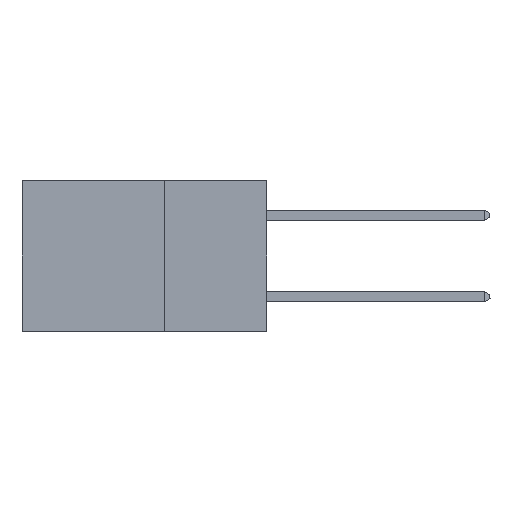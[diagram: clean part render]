
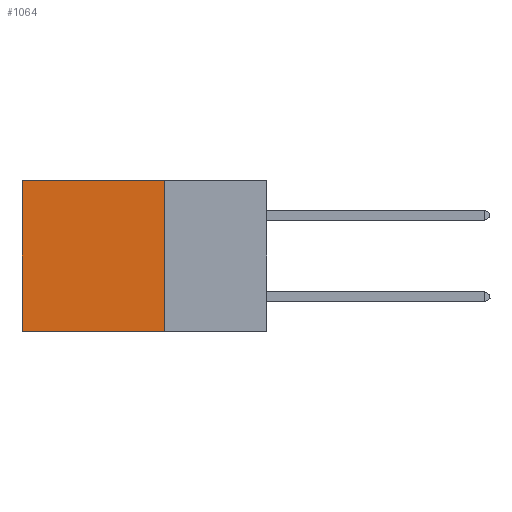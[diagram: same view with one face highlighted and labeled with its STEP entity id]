
A CAD part, left-side view. The second image highlights one B-rep face of the part: STEP entity #1064.
In plain terms, the highlighted planar face has unit normal (-1, 0, 0).
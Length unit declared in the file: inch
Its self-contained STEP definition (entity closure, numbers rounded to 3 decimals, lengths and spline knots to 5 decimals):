
#1064 = ADVANCED_FACE ( 'NONE', ( #12632 ), #14501, .F. ) ;
#1377 = ORIENTED_EDGE ( 'NONE', *, *, #7492, .T. ) ;
#2308 = DIRECTION ( 'NONE',  ( 0., 0., -1. ) ) ;
#2912 = CARTESIAN_POINT ( 'NONE',  ( 0.2875, 0.6, 0. ) ) ;
#4294 = DIRECTION ( 'NONE',  ( 0., 1., 0. ) ) ;
#4719 = VECTOR ( 'NONE', #12268, 39.37008 ) ;
#5949 = CARTESIAN_POINT ( 'NONE',  ( 0.2875, 0.25, -0.37 ) ) ;
#7492 = EDGE_CURVE ( 'NONE', #18256, #28915, #10440, .T. ) ;
#8847 = CARTESIAN_POINT ( 'NONE',  ( 0.2875, 0.6, 0. ) ) ;
#9198 = VERTEX_POINT ( 'NONE', #5949 ) ;
#9923 = EDGE_CURVE ( 'NONE', #9198, #11250, #27934, .T. ) ;
#10440 = LINE ( 'NONE', #22152, #19421 ) ;
#11250 = VERTEX_POINT ( 'NONE', #20444 ) ;
#12070 = ORIENTED_EDGE ( 'NONE', *, *, #9923, .F. ) ;
#12263 = CARTESIAN_POINT ( 'NONE',  ( 0.2875, 0.25, 0. ) ) ;
#12268 = DIRECTION ( 'NONE',  ( 0., 0., -1. ) ) ;
#12632 = FACE_OUTER_BOUND ( 'NONE', #24332, .T. ) ;
#12820 = CARTESIAN_POINT ( 'NONE',  ( 0.2875, 0.25, 0. ) ) ;
#13550 = LINE ( 'NONE', #12820, #29356 ) ;
#13733 = LINE ( 'NONE', #2912, #4719 ) ;
#13765 = EDGE_CURVE ( 'NONE', #28915, #11250, #13733, .T. ) ;
#14501 = PLANE ( 'NONE',  #23375 ) ;
#15101 = CARTESIAN_POINT ( 'NONE',  ( 0.2875, 0.25, 0. ) ) ;
#15750 = VECTOR ( 'NONE', #4294, 39.37008 ) ;
#17847 = DIRECTION ( 'NONE',  ( 0., 0., -1. ) ) ;
#18256 = VERTEX_POINT ( 'NONE', #15101 ) ;
#19421 = VECTOR ( 'NONE', #26770, 39.37008 ) ;
#20444 = CARTESIAN_POINT ( 'NONE',  ( 0.2875, 0.6, -0.37 ) ) ;
#22152 = CARTESIAN_POINT ( 'NONE',  ( 0.2875, 0.25, 0. ) ) ;
#23006 = EDGE_CURVE ( 'NONE', #18256, #9198, #13550, .T. ) ;
#23375 = AXIS2_PLACEMENT_3D ( 'NONE', #12263, #29512, #2308 ) ;
#23475 = ORIENTED_EDGE ( 'NONE', *, *, #23006, .F. ) ;
#24332 = EDGE_LOOP ( 'NONE', ( #26594, #12070, #23475, #1377 ) ) ;
#24517 = CARTESIAN_POINT ( 'NONE',  ( 0.2875, 0.25, -0.37 ) ) ;
#26594 = ORIENTED_EDGE ( 'NONE', *, *, #13765, .T. ) ;
#26770 = DIRECTION ( 'NONE',  ( 0., 1., 0. ) ) ;
#27934 = LINE ( 'NONE', #24517, #15750 ) ;
#28915 = VERTEX_POINT ( 'NONE', #8847 ) ;
#29356 = VECTOR ( 'NONE', #17847, 39.37008 ) ;
#29512 = DIRECTION ( 'NONE',  ( 1., 0., 0. ) ) ;
